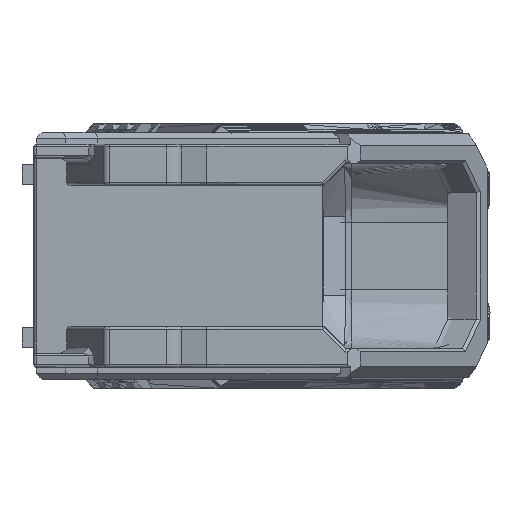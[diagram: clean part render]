
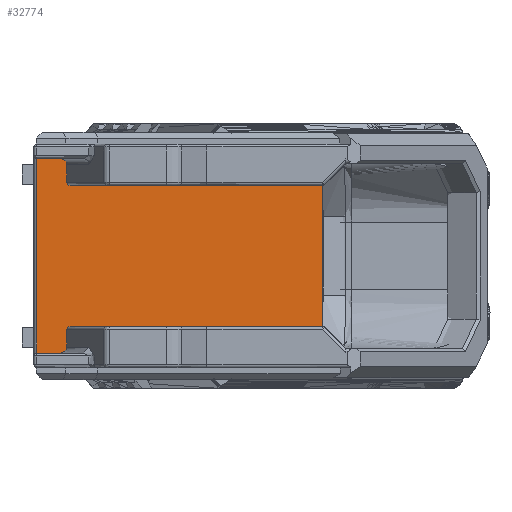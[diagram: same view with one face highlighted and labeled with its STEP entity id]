
A CAD part, left-side view. The second image highlights one B-rep face of the part: STEP entity #32774.
In plain terms, the highlighted planar face has unit normal (-1, 0, 0).
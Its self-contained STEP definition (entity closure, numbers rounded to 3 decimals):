
#159=ELLIPSE('',#35011,0.577,0.5);
#160=ELLIPSE('',#35013,0.577,0.5);
#162=ELLIPSE('',#35029,1.155,1.);
#163=ELLIPSE('',#35040,1.155,1.);
#648=CIRCLE('',#35166,0.5);
#649=CIRCLE('',#35167,0.5);
#896=FACE_OUTER_BOUND('',#3192,.T.);
#3192=EDGE_LOOP('',(#22064,#22065,#22066,#22067,#22068,#22069,#22070,#22071,
#22072,#22073,#22074,#22075,#22076,#22077,#22078,#22079));
#5467=LINE('',#48085,#9746);
#5476=LINE('',#48119,#9755);
#5493=LINE('',#48182,#9772);
#5514=LINE('',#48416,#9793);
#5516=LINE('',#48492,#9795);
#5563=LINE('',#49007,#9842);
#5629=LINE('',#49743,#9908);
#5634=LINE('',#49757,#9913);
#5635=LINE('',#49760,#9914);
#5636=LINE('',#49762,#9915);
#9746=VECTOR('',#37743,1000.);
#9755=VECTOR('',#37776,1000.);
#9772=VECTOR('',#37829,1000.);
#9793=VECTOR('',#37942,1000.);
#9795=VECTOR('',#37954,1000.);
#9842=VECTOR('',#38165,1000.);
#9908=VECTOR('',#38321,1000.);
#9913=VECTOR('',#38338,1000.);
#9914=VECTOR('',#38341,1000.);
#9915=VECTOR('',#38342,1000.);
#13868=VERTEX_POINT('',#46743);
#14018=VERTEX_POINT('',#48082);
#14019=VERTEX_POINT('',#48084);
#14031=VERTEX_POINT('',#48116);
#14032=VERTEX_POINT('',#48118);
#14052=VERTEX_POINT('',#48178);
#14054=VERTEX_POINT('',#48181);
#14073=VERTEX_POINT('',#48294);
#14074=VERTEX_POINT('',#48298);
#14085=VERTEX_POINT('',#48414);
#14086=VERTEX_POINT('',#48488);
#14088=VERTEX_POINT('',#48491);
#14197=VERTEX_POINT('',#49740);
#14201=VERTEX_POINT('',#49756);
#14202=VERTEX_POINT('',#49758);
#14203=VERTEX_POINT('',#49761);
#16549=EDGE_CURVE('',#14019,#14018,#5467,.T.);
#16565=EDGE_CURVE('',#14032,#14031,#5476,.T.);
#16593=EDGE_CURVE('',#14054,#14052,#5493,.T.);
#16626=EDGE_CURVE('',#14054,#14073,#159,.T.);
#16628=EDGE_CURVE('',#14074,#14031,#160,.T.);
#16649=EDGE_CURVE('',#13868,#14085,#5514,.T.);
#16650=EDGE_CURVE('',#14052,#14085,#162,.T.);
#16655=EDGE_CURVE('',#14086,#14088,#5516,.T.);
#16669=EDGE_CURVE('',#14086,#14032,#163,.T.);
#16759=EDGE_CURVE('',#14088,#13868,#5563,.T.);
#16860=EDGE_CURVE('',#14197,#14074,#5629,.T.);
#16867=EDGE_CURVE('',#14073,#14201,#5634,.T.);
#16868=EDGE_CURVE('',#14202,#14197,#648,.T.);
#16869=EDGE_CURVE('',#14019,#14202,#5635,.T.);
#16870=EDGE_CURVE('',#14203,#14018,#5636,.T.);
#16871=EDGE_CURVE('',#14201,#14203,#649,.T.);
#22064=ORIENTED_EDGE('',*,*,#16867,.F.);
#22065=ORIENTED_EDGE('',*,*,#16626,.F.);
#22066=ORIENTED_EDGE('',*,*,#16593,.T.);
#22067=ORIENTED_EDGE('',*,*,#16650,.T.);
#22068=ORIENTED_EDGE('',*,*,#16649,.F.);
#22069=ORIENTED_EDGE('',*,*,#16759,.F.);
#22070=ORIENTED_EDGE('',*,*,#16655,.F.);
#22071=ORIENTED_EDGE('',*,*,#16669,.T.);
#22072=ORIENTED_EDGE('',*,*,#16565,.T.);
#22073=ORIENTED_EDGE('',*,*,#16628,.F.);
#22074=ORIENTED_EDGE('',*,*,#16860,.F.);
#22075=ORIENTED_EDGE('',*,*,#16868,.F.);
#22076=ORIENTED_EDGE('',*,*,#16869,.F.);
#22077=ORIENTED_EDGE('',*,*,#16549,.T.);
#22078=ORIENTED_EDGE('',*,*,#16870,.F.);
#22079=ORIENTED_EDGE('',*,*,#16871,.F.);
#30523=PLANE('',#35165);
#32774=ADVANCED_FACE('',(#896),#30523,.F.);
#35011=AXIS2_PLACEMENT_3D('',#48295,#37898,#37899);
#35013=AXIS2_PLACEMENT_3D('',#48299,#37903,#37904);
#35029=AXIS2_PLACEMENT_3D('',#48418,#37945,#37946);
#35040=AXIS2_PLACEMENT_3D('',#48628,#37975,#37976);
#35165=AXIS2_PLACEMENT_3D('',#49755,#38336,#38337);
#35166=AXIS2_PLACEMENT_3D('',#49759,#38339,#38340);
#35167=AXIS2_PLACEMENT_3D('',#49763,#38343,#38344);
#37743=DIRECTION('',(0.,0.,1.));
#37776=DIRECTION('',(0.,0.,1.));
#37829=DIRECTION('',(0.,0.,1.));
#37898=DIRECTION('center_axis',(-1.,0.,0.));
#37899=DIRECTION('ref_axis',(0.,1.,0.));
#37903=DIRECTION('center_axis',(-1.,0.,0.));
#37904=DIRECTION('ref_axis',(0.,1.,0.));
#37942=DIRECTION('',(0.,-1.,0.));
#37945=DIRECTION('center_axis',(-1.,0.,0.));
#37946=DIRECTION('ref_axis',(0.,1.,0.));
#37954=DIRECTION('',(0.,1.,0.));
#37975=DIRECTION('center_axis',(-1.,0.,0.));
#37976=DIRECTION('ref_axis',(0.,1.,0.));
#38165=DIRECTION('',(0.,0.,1.));
#38321=DIRECTION('',(0.,1.,0.));
#38336=DIRECTION('center_axis',(1.,0.,0.));
#38337=DIRECTION('ref_axis',(0.,0.,
-1.));
#38338=DIRECTION('',(0.,-1.,0.));
#38339=DIRECTION('center_axis',(-1.,0.,0.));
#38340=DIRECTION('ref_axis',(0.,-0.383,0.924));
#38341=DIRECTION('',(0.,-0.707,-0.707));
#38342=DIRECTION('',(0.,0.707,-0.707));
#38343=DIRECTION('center_axis',(-1.,0.,0.));
#38344=DIRECTION('ref_axis',(0.,-0.383,-0.924));
#46743=CARTESIAN_POINT('',(-82.4,-8.79,17.5));
#48082=CARTESIAN_POINT('',(-82.4,-57.29,12.75));
#48084=CARTESIAN_POINT('',(-82.4,-57.29,-10.75));
#48085=CARTESIAN_POINT('',(-82.4,-57.29,9.17));
#48116=CARTESIAN_POINT('',(-82.4,-13.907,-11.5));
#48118=CARTESIAN_POINT('',(-82.4,-13.907,-14.5));
#48119=CARTESIAN_POINT('',(-82.4,-13.907,-9.1));
#48178=CARTESIAN_POINT('',(-82.4,-13.907,16.5));
#48181=CARTESIAN_POINT('',(-82.4,-13.907,13.5));
#48182=CARTESIAN_POINT('',(-82.4,-13.907,-9.1));
#48294=CARTESIAN_POINT('',(-82.4,-14.485,13.));
#48295=CARTESIAN_POINT('Origin',(-82.4,-14.485,13.5));
#48298=CARTESIAN_POINT('',(-82.4,-14.485,-11.));
#48299=CARTESIAN_POINT('Origin',(-82.4,-14.485,-11.5));
#48414=CARTESIAN_POINT('',(-82.4,-12.753,17.5));
#48416=CARTESIAN_POINT('',(-82.4,-32.84,17.5));
#48418=CARTESIAN_POINT('Origin',(-82.4,-12.753,16.5));
#48488=CARTESIAN_POINT('',(-82.4,-12.753,-15.5));
#48491=CARTESIAN_POINT('',(-82.4,-8.79,-15.5));
#48492=CARTESIAN_POINT('',(-82.4,-31.547,-15.5));
#48628=CARTESIAN_POINT('Origin',(-82.4,-12.753,-14.5));
#49007=CARTESIAN_POINT('',(-82.4,-8.79,1.));
#49740=CARTESIAN_POINT('',(-82.4,-57.332,-11.));
#49743=CARTESIAN_POINT('',(-82.4,-31.547,-11.));
#49755=CARTESIAN_POINT('Origin',(-82.4,-31.141,1.));
#49756=CARTESIAN_POINT('',(-82.4,-57.333,13.));
#49757=CARTESIAN_POINT('',(-82.4,-32.84,13.));
#49758=CARTESIAN_POINT('',(-82.4,-57.686,-11.146));
#49759=CARTESIAN_POINT('Origin',(-82.4,-57.332,-11.5));
#49760=CARTESIAN_POINT('',(-82.4,-48.815,-2.275));
#49761=CARTESIAN_POINT('',(-82.4,-57.686,13.146));
#49762=CARTESIAN_POINT('',(-82.4,-48.815,4.275));
#49763=CARTESIAN_POINT('Origin',(-82.4,-57.333,13.5));
